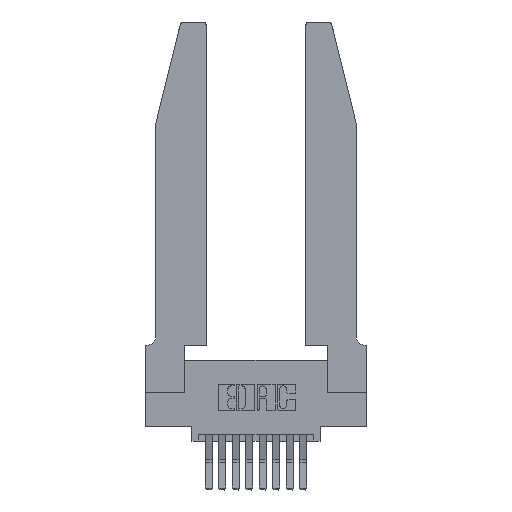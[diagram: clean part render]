
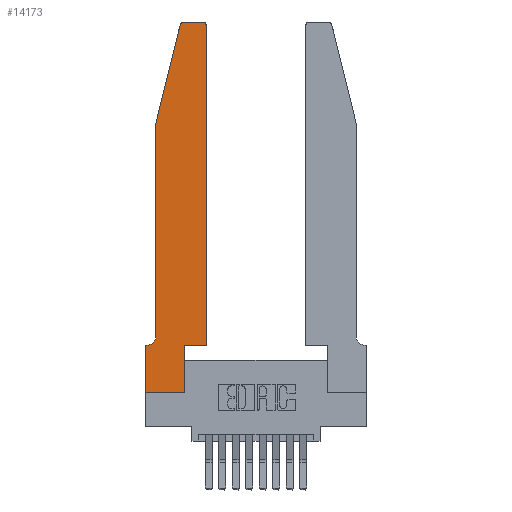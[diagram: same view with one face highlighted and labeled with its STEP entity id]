
A CAD part, top view. The second image highlights one B-rep face of the part: STEP entity #14173.
In plain terms, the highlighted planar face has unit normal (0, 0, 1).
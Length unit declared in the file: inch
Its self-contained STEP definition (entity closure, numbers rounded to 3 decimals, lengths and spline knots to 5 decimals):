
#497 = LINE ( 'NONE', #7763, #9962 ) ;
#517 = CARTESIAN_POINT ( 'NONE',  ( 0.0755, 0.42, 0.37 ) ) ;
#714 = CARTESIAN_POINT ( 'NONE',  ( 0.4505, 0.35, 0.37 ) ) ;
#932 = EDGE_CURVE ( 'NONE', #12094, #7917, #8069, .T. ) ;
#1176 = CARTESIAN_POINT ( 'NONE',  ( 0.2865, 0.35, 0.37 ) ) ;
#1373 = CARTESIAN_POINT ( 'NONE',  ( 0., 0., 0.37 ) ) ;
#1399 = VERTEX_POINT ( 'NONE', #14801 ) ;
#1444 = FACE_OUTER_BOUND ( 'NONE', #11782, .T. ) ;
#1479 = EDGE_CURVE ( 'NONE', #2241, #9038, #10532, .T. ) ;
#1704 = ORIENTED_EDGE ( 'NONE', *, *, #932, .T. ) ;
#1774 = PLANE ( 'NONE',  #7827 ) ;
#2223 = CARTESIAN_POINT ( 'NONE',  ( 0.0055, 0.35, 0.37 ) ) ;
#2241 = VERTEX_POINT ( 'NONE', #1373 ) ;
#2442 = LINE ( 'NONE', #10947, #8596 ) ;
#2561 = ORIENTED_EDGE ( 'NONE', *, *, #10131, .T. ) ;
#2830 = ORIENTED_EDGE ( 'NONE', *, *, #1479, .T. ) ;
#2989 = DIRECTION ( 'NONE',  ( 0., -1., 0. ) ) ;
#3030 = CARTESIAN_POINT ( 'NONE',  ( 0., 0.35, 0.37 ) ) ;
#3111 = CARTESIAN_POINT ( 'NONE',  ( 0.0755, 2., 0.37 ) ) ;
#3461 = CARTESIAN_POINT ( 'NONE',  ( 0.4505, 0.35, 0.37 ) ) ;
#3487 = CIRCLE ( 'NONE', #9732, 0.03 ) ;
#3860 = DIRECTION ( 'NONE',  ( 0., 0., 1. ) ) ;
#3972 = ORIENTED_EDGE ( 'NONE', *, *, #15185, .T. ) ;
#3999 = LINE ( 'NONE', #1176, #15779 ) ;
#4055 = CARTESIAN_POINT ( 'NONE',  ( 0.2865, 0., 0.37 ) ) ;
#4266 = DIRECTION ( 'NONE',  ( 0., 0., 1. ) ) ;
#4439 = CIRCLE ( 'NONE', #9937, 0.07 ) ;
#4800 = VECTOR ( 'NONE', #10265, 39.37008 ) ;
#4803 = ORIENTED_EDGE ( 'NONE', *, *, #15726, .T. ) ;
#5078 = CARTESIAN_POINT ( 'NONE',  ( 0.0055, 0.42, 0.37 ) ) ;
#5143 = CARTESIAN_POINT ( 'NONE',  ( 0.4205, 2.75, 0.37 ) ) ;
#6194 = DIRECTION ( 'NONE',  ( -0.239, -0.971, 0. ) ) ;
#6235 = CARTESIAN_POINT ( 'NONE',  ( 0.4505, 2.72, 0.37 ) ) ;
#6286 = DIRECTION ( 'NONE',  ( -1., 0., 0. ) ) ;
#6306 = DIRECTION ( 'NONE',  ( 0., 0., 1. ) ) ;
#6443 = VERTEX_POINT ( 'NONE', #714 ) ;
#6792 = VECTOR ( 'NONE', #13255, 39.37008 ) ;
#6802 = CARTESIAN_POINT ( 'NONE',  ( 0., 0., 0.37 ) ) ;
#7263 = VECTOR ( 'NONE', #10229, 39.37008 ) ;
#7302 = VERTEX_POINT ( 'NONE', #6235 ) ;
#7303 = DIRECTION ( 'NONE',  ( 1., 0., 0. ) ) ;
#7672 = EDGE_CURVE ( 'NONE', #15704, #6443, #2442, .T. ) ;
#7763 = CARTESIAN_POINT ( 'NONE',  ( 0.2605, 2.75, 0.37 ) ) ;
#7827 = AXIS2_PLACEMENT_3D ( 'NONE', #3030, #4266, #12780 ) ;
#7917 = VERTEX_POINT ( 'NONE', #14980 ) ;
#7990 = LINE ( 'NONE', #12288, #10848 ) ;
#8069 = LINE ( 'NONE', #10296, #4800 ) ;
#8081 = ORIENTED_EDGE ( 'NONE', *, *, #12988, .T. ) ;
#8138 = ORIENTED_EDGE ( 'NONE', *, *, #7672, .T. ) ;
#8381 = VERTEX_POINT ( 'NONE', #9924 ) ;
#8420 = CARTESIAN_POINT ( 'NONE',  ( 0.2865, 0.35, 0.37 ) ) ;
#8437 = VERTEX_POINT ( 'NONE', #5143 ) ;
#8536 = DIRECTION ( 'NONE',  ( 0., 1., 0. ) ) ;
#8596 = VECTOR ( 'NONE', #7303, 39.37008 ) ;
#8931 = CARTESIAN_POINT ( 'NONE',  ( 0.284, 2.75, 0.37 ) ) ;
#9038 = VERTEX_POINT ( 'NONE', #4055 ) ;
#9039 = LINE ( 'NONE', #3111, #12613 ) ;
#9120 = DIRECTION ( 'NONE',  ( -1., 0., 0. ) ) ;
#9692 = ORIENTED_EDGE ( 'NONE', *, *, #13602, .T. ) ;
#9732 = AXIS2_PLACEMENT_3D ( 'NONE', #13594, #6306, #14818 ) ;
#9848 = ORIENTED_EDGE ( 'NONE', *, *, #13859, .T. ) ;
#9924 = CARTESIAN_POINT ( 'NONE',  ( 0.0755, 2., 0.37 ) ) ;
#9937 = AXIS2_PLACEMENT_3D ( 'NONE', #5078, #13579, #6286 ) ;
#9962 = VECTOR ( 'NONE', #9120, 39.37008 ) ;
#10066 = LINE ( 'NONE', #3461, #6792 ) ;
#10131 = EDGE_CURVE ( 'NONE', #11107, #1399, #12112, .T. ) ;
#10229 = DIRECTION ( 'NONE',  ( 1., 0., 0. ) ) ;
#10265 = DIRECTION ( 'NONE',  ( -1., 0., 0. ) ) ;
#10296 = CARTESIAN_POINT ( 'NONE',  ( 0.0755, 0.35, 0.37 ) ) ;
#10336 = CARTESIAN_POINT ( 'NONE',  ( 0., 0., 0.37 ) ) ;
#10434 = ORIENTED_EDGE ( 'NONE', *, *, #11022, .T. ) ;
#10532 = LINE ( 'NONE', #6802, #7263 ) ;
#10848 = VECTOR ( 'NONE', #6194, 39.37008 ) ;
#10852 = ORIENTED_EDGE ( 'NONE', *, *, #11667, .T. ) ;
#10947 = CARTESIAN_POINT ( 'NONE',  ( 0.4505, 0.35, 0.37 ) ) ;
#11022 = EDGE_CURVE ( 'NONE', #7302, #8437, #3487, .T. ) ;
#11033 = VECTOR ( 'NONE', #2989, 39.37008 ) ;
#11107 = VERTEX_POINT ( 'NONE', #8931 ) ;
#11178 = CARTESIAN_POINT ( 'NONE',  ( 0.284, 2.72, 0.37 ) ) ;
#11667 = EDGE_CURVE ( 'NONE', #15493, #12094, #4439, .T. ) ;
#11673 = DIRECTION ( 'NONE',  ( 0., -1., 0. ) ) ;
#11782 = EDGE_LOOP ( 'NONE', ( #9692, #2561, #3972, #8081, #10852, #1704, #13750, #2830, #9848, #8138, #4803, #10434 ) ) ;
#12094 = VERTEX_POINT ( 'NONE', #2223 ) ;
#12112 = CIRCLE ( 'NONE', #12233, 0.03 ) ;
#12233 = AXIS2_PLACEMENT_3D ( 'NONE', #11178, #3860, #12391 ) ;
#12288 = CARTESIAN_POINT ( 'NONE',  ( 0.0755, 2., 0.37 ) ) ;
#12391 = DIRECTION ( 'NONE',  ( 1., 0., 0. ) ) ;
#12613 = VECTOR ( 'NONE', #11673, 39.37008 ) ;
#12780 = DIRECTION ( 'NONE',  ( 1., 0., 0. ) ) ;
#12988 = EDGE_CURVE ( 'NONE', #8381, #15493, #9039, .T. ) ;
#13255 = DIRECTION ( 'NONE',  ( 0., 1., 0. ) ) ;
#13579 = DIRECTION ( 'NONE',  ( 0., 0., -1. ) ) ;
#13594 = CARTESIAN_POINT ( 'NONE',  ( 0.4205, 2.72, 0.37 ) ) ;
#13602 = EDGE_CURVE ( 'NONE', #8437, #11107, #497, .T. ) ;
#13750 = ORIENTED_EDGE ( 'NONE', *, *, #15444, .T. ) ;
#13859 = EDGE_CURVE ( 'NONE', #9038, #15704, #3999, .T. ) ;
#14173 = ADVANCED_FACE ( 'NONE', ( #1444 ), #1774, .T. ) ;
#14220 = LINE ( 'NONE', #10336, #11033 ) ;
#14801 = CARTESIAN_POINT ( 'NONE',  ( 0.25487, 2.72718, 0.37 ) ) ;
#14818 = DIRECTION ( 'NONE',  ( 1., 0., 0. ) ) ;
#14980 = CARTESIAN_POINT ( 'NONE',  ( 0., 0.35, 0.37 ) ) ;
#15185 = EDGE_CURVE ( 'NONE', #1399, #8381, #7990, .T. ) ;
#15444 = EDGE_CURVE ( 'NONE', #7917, #2241, #14220, .T. ) ;
#15493 = VERTEX_POINT ( 'NONE', #517 ) ;
#15704 = VERTEX_POINT ( 'NONE', #8420 ) ;
#15726 = EDGE_CURVE ( 'NONE', #6443, #7302, #10066, .T. ) ;
#15779 = VECTOR ( 'NONE', #8536, 39.37008 ) ;
